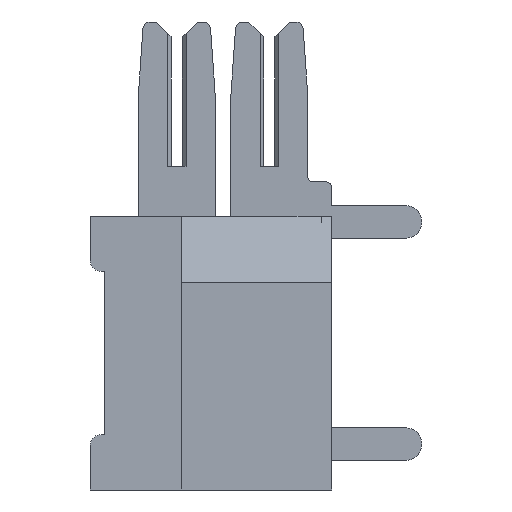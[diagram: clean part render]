
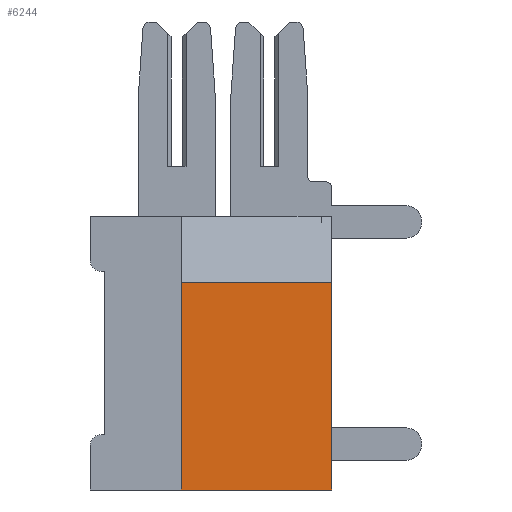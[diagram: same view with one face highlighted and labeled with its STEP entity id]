
A CAD part, left-side view. The second image highlights one B-rep face of the part: STEP entity #6244.
In plain terms, the highlighted planar face has unit normal (-1, 0, 0).
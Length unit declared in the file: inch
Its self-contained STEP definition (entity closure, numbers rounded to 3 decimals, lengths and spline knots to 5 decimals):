
#46 = ORIENTED_EDGE ( 'NONE', *, *, #6109, .T. ) ;
#379 = CARTESIAN_POINT ( 'NONE',  ( 0., 0.203, -0.37 ) ) ;
#614 = FACE_OUTER_BOUND ( 'NONE', #5648, .T. ) ;
#763 = CARTESIAN_POINT ( 'NONE',  ( 0., 0.326, -0.37 ) ) ;
#1096 = DIRECTION ( 'NONE',  ( 0., 0., 1. ) ) ;
#1471 = VECTOR ( 'NONE', #1096, 39.37008 ) ;
#1573 = LINE ( 'NONE', #379, #1471 ) ;
#1590 = DIRECTION ( 'NONE',  ( 1., 0., 0. ) ) ;
#1631 = VERTEX_POINT ( 'NONE', #6249 ) ;
#2135 = EDGE_CURVE ( 'NONE', #7466, #8289, #1573, .T. ) ;
#2240 = CARTESIAN_POINT ( 'NONE',  ( 0., 0.203, -0.37 ) ) ;
#2263 = PLANE ( 'NONE',  #5951 ) ;
#2293 = ORIENTED_EDGE ( 'NONE', *, *, #2135, .F. ) ;
#2422 = CARTESIAN_POINT ( 'NONE',  ( 0., 0.203, -0.09 ) ) ;
#2487 = CARTESIAN_POINT ( 'NONE',  ( 0., 0., 0. ) ) ;
#3345 = CARTESIAN_POINT ( 'NONE',  ( 0., 0., -0.37 ) ) ;
#3533 = DIRECTION ( 'NONE',  ( 0., 0., -1. ) ) ;
#4460 = LINE ( 'NONE', #2487, #8169 ) ;
#4587 = CARTESIAN_POINT ( 'NONE',  ( 0., 0., -0.09 ) ) ;
#4950 = EDGE_CURVE ( 'NONE', #7141, #1631, #4460, .T. ) ;
#5158 = EDGE_CURVE ( 'NONE', #1631, #8289, #5753, .T. ) ;
#5275 = DIRECTION ( 'NONE',  ( 0., 1., 0. ) ) ;
#5483 = DIRECTION ( 'NONE',  ( 0., 0., 1. ) ) ;
#5648 = EDGE_LOOP ( 'NONE', ( #6638, #7195, #2293, #46 ) ) ;
#5753 = LINE ( 'NONE', #4587, #7668 ) ;
#5951 = AXIS2_PLACEMENT_3D ( 'NONE', #8066, #1590, #3533 ) ;
#5953 = DIRECTION ( 'NONE',  ( 0., -1., 0. ) ) ;
#6109 = EDGE_CURVE ( 'NONE', #7466, #7141, #7811, .T. ) ;
#6244 = ADVANCED_FACE ( 'NONE', ( #614 ), #2263, .F. ) ;
#6249 = CARTESIAN_POINT ( 'NONE',  ( 0., 0., -0.09 ) ) ;
#6638 = ORIENTED_EDGE ( 'NONE', *, *, #4950, .T. ) ;
#6712 = VECTOR ( 'NONE', #5953, 39.37008 ) ;
#7141 = VERTEX_POINT ( 'NONE', #3345 ) ;
#7195 = ORIENTED_EDGE ( 'NONE', *, *, #5158, .T. ) ;
#7466 = VERTEX_POINT ( 'NONE', #2240 ) ;
#7668 = VECTOR ( 'NONE', #5275, 39.37008 ) ;
#7811 = LINE ( 'NONE', #763, #6712 ) ;
#8066 = CARTESIAN_POINT ( 'NONE',  ( 0., 0.326, 0. ) ) ;
#8169 = VECTOR ( 'NONE', #5483, 39.37008 ) ;
#8289 = VERTEX_POINT ( 'NONE', #2422 ) ;
